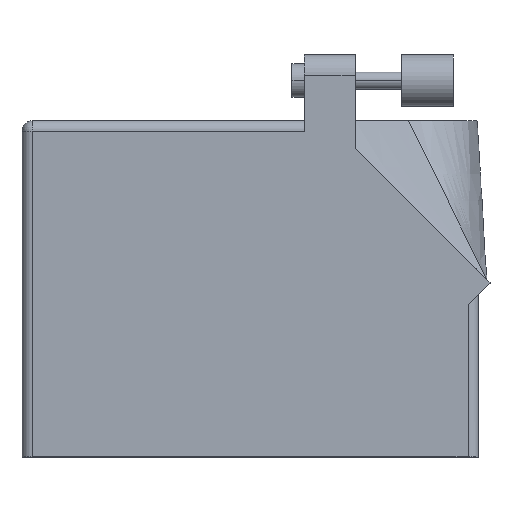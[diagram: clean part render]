
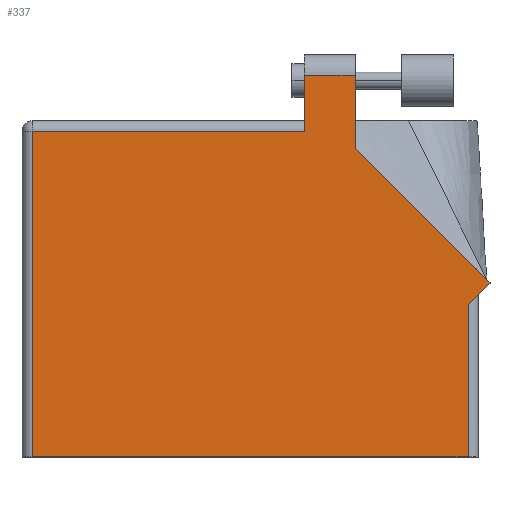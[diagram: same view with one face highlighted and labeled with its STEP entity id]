
A CAD part, top view. The second image highlights one B-rep face of the part: STEP entity #337.
In plain terms, the highlighted planar face has unit normal (0, 0, 1).
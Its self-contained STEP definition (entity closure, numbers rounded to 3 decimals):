
#94 = LINE ( 'NONE', #493, #2332 ) ;
#139 = VECTOR ( 'NONE', #543, 1000. ) ;
#152 = CARTESIAN_POINT ( 'NONE',  ( 71.773, 26.688, 0. ) ) ;
#159 = DIRECTION ( 'NONE',  ( 0., -1., 0. ) ) ;
#198 = VERTEX_POINT ( 'NONE', #1185 ) ;
#212 = LINE ( 'NONE', #825, #646 ) ;
#337 = ADVANCED_FACE ( 'NONE', ( #1074 ), #1846, .F. ) ;
#342 = EDGE_CURVE ( 'NONE', #664, #198, #94, .T. ) ;
#440 = VECTOR ( 'NONE', #2174, 1000. ) ;
#444 = VERTEX_POINT ( 'NONE', #152 ) ;
#464 = VERTEX_POINT ( 'NONE', #739 ) ;
#468 = EDGE_LOOP ( 'NONE', ( #1072, #2234, #1842, #1725, #505, #772, #2168, #1157, #987 ) ) ;
#489 = VERTEX_POINT ( 'NONE', #1309 ) ;
#493 = CARTESIAN_POINT ( 'NONE',  ( 0., 49.987, 0. ) ) ;
#494 = EDGE_CURVE ( 'NONE', #2485, #444, #750, .T. ) ;
#505 = ORIENTED_EDGE ( 'NONE', *, *, #517, .T. ) ;
#517 = EDGE_CURVE ( 'NONE', #198, #2452, #1908, .T. ) ;
#543 = DIRECTION ( 'NONE',  ( 0.707, 0.707, 0. ) ) ;
#646 = VECTOR ( 'NONE', #1432, 1000. ) ;
#664 = VERTEX_POINT ( 'NONE', #1203 ) ;
#696 = DIRECTION ( 'NONE',  ( -1., 0., 0. ) ) ;
#698 = CARTESIAN_POINT ( 'NONE',  ( 68.402, 23.317, 0. ) ) ;
#739 = CARTESIAN_POINT ( 'NONE',  ( 51.105, 58.547, 0. ) ) ;
#750 = LINE ( 'NONE', #1927, #139 ) ;
#772 = ORIENTED_EDGE ( 'NONE', *, *, #1870, .T. ) ;
#785 = EDGE_CURVE ( 'NONE', #489, #464, #1391, .T. ) ;
#795 = EDGE_CURVE ( 'NONE', #1121, #2485, #1645, .T. ) ;
#825 = CARTESIAN_POINT ( 'NONE',  ( 0., 0., 0. ) ) ;
#846 = VECTOR ( 'NONE', #1302, 1000. ) ;
#894 = DIRECTION ( 'NONE',  ( -1., 0., 0. ) ) ;
#958 = VECTOR ( 'NONE', #159, 1000. ) ;
#987 = ORIENTED_EDGE ( 'NONE', *, *, #1769, .T. ) ;
#989 = CARTESIAN_POINT ( 'NONE',  ( 51.105, 47.356, 0. ) ) ;
#1072 = ORIENTED_EDGE ( 'NONE', *, *, #785, .T. ) ;
#1074 = FACE_OUTER_BOUND ( 'NONE', #468, .T. ) ;
#1101 = EDGE_CURVE ( 'NONE', #1326, #664, #2393, .T. ) ;
#1121 = VERTEX_POINT ( 'NONE', #2269 ) ;
#1157 = ORIENTED_EDGE ( 'NONE', *, *, #494, .T. ) ;
#1185 = CARTESIAN_POINT ( 'NONE',  ( 1.575, 49.987, 0. ) ) ;
#1203 = CARTESIAN_POINT ( 'NONE',  ( 43.307, 49.987, 0. ) ) ;
#1301 = CARTESIAN_POINT ( 'NONE',  ( 0., 51.562, 0. ) ) ;
#1302 = DIRECTION ( 'NONE',  ( -1., 0., 0. ) ) ;
#1304 = CARTESIAN_POINT ( 'NONE',  ( 1.575, 0., 0. ) ) ;
#1309 = CARTESIAN_POINT ( 'NONE',  ( 51.105, 47.356, 0. ) ) ;
#1326 = VERTEX_POINT ( 'NONE', #2322 ) ;
#1391 = LINE ( 'NONE', #989, #1561 ) ;
#1432 = DIRECTION ( 'NONE',  ( 1., 0., 0. ) ) ;
#1452 = VECTOR ( 'NONE', #1815, 1000. ) ;
#1481 = CARTESIAN_POINT ( 'NONE',  ( 1.575, 0., 0. ) ) ;
#1502 = LINE ( 'NONE', #1675, #846 ) ;
#1520 = EDGE_CURVE ( 'NONE', #464, #1326, #1502, .T. ) ;
#1561 = VECTOR ( 'NONE', #2163, 1000. ) ;
#1645 = LINE ( 'NONE', #2434, #1452 ) ;
#1675 = CARTESIAN_POINT ( 'NONE',  ( 43.307, 58.547, 0. ) ) ;
#1725 = ORIENTED_EDGE ( 'NONE', *, *, #342, .T. ) ;
#1750 = DIRECTION ( 'NONE',  ( 0., -1., 0. ) ) ;
#1769 = EDGE_CURVE ( 'NONE', #444, #489, #1942, .T. ) ;
#1815 = DIRECTION ( 'NONE',  ( 0., 1., 0. ) ) ;
#1842 = ORIENTED_EDGE ( 'NONE', *, *, #1101, .T. ) ;
#1846 = PLANE ( 'NONE',  #1973 ) ;
#1870 = EDGE_CURVE ( 'NONE', #2452, #1121, #212, .T. ) ;
#1908 = LINE ( 'NONE', #1304, #958 ) ;
#1927 = CARTESIAN_POINT ( 'NONE',  ( 69.977, 24.892, 0. ) ) ;
#1942 = LINE ( 'NONE', #2515, #440 ) ;
#1973 = AXIS2_PLACEMENT_3D ( 'NONE', #1301, #2416, #696 ) ;
#1990 = VECTOR ( 'NONE', #1750, 1000. ) ;
#2017 = CARTESIAN_POINT ( 'NONE',  ( 43.307, 51.562, 0. ) ) ;
#2163 = DIRECTION ( 'NONE',  ( 0., 1., 0. ) ) ;
#2168 = ORIENTED_EDGE ( 'NONE', *, *, #795, .T. ) ;
#2174 = DIRECTION ( 'NONE',  ( -0.707, 0.707, 0. ) ) ;
#2234 = ORIENTED_EDGE ( 'NONE', *, *, #1520, .T. ) ;
#2269 = CARTESIAN_POINT ( 'NONE',  ( 68.402, 0., 0. ) ) ;
#2322 = CARTESIAN_POINT ( 'NONE',  ( 43.307, 58.547, 0. ) ) ;
#2332 = VECTOR ( 'NONE', #894, 1000. ) ;
#2393 = LINE ( 'NONE', #2017, #1990 ) ;
#2416 = DIRECTION ( 'NONE',  ( 0., 0., -1. ) ) ;
#2434 = CARTESIAN_POINT ( 'NONE',  ( 68.402, 24.892, 0. ) ) ;
#2452 = VERTEX_POINT ( 'NONE', #1481 ) ;
#2485 = VERTEX_POINT ( 'NONE', #698 ) ;
#2515 = CARTESIAN_POINT ( 'NONE',  ( 71.773, 26.688, 0. ) ) ;
